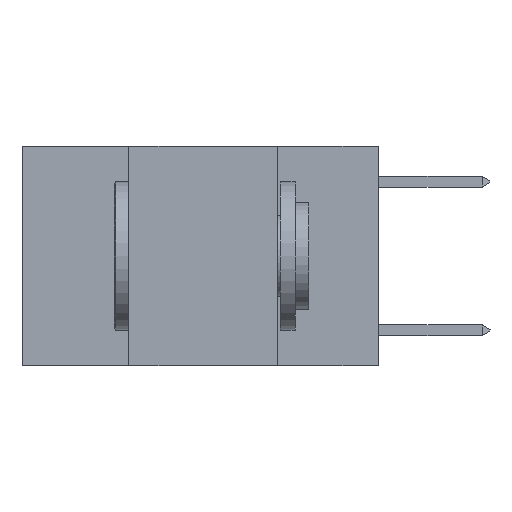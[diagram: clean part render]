
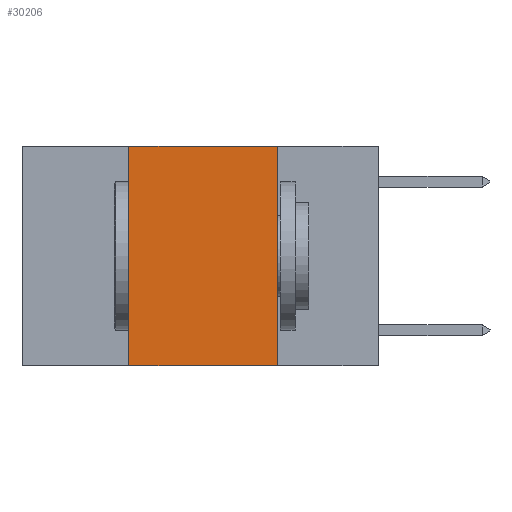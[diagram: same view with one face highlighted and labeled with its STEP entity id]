
A CAD part, left-side view. The second image highlights one B-rep face of the part: STEP entity #30206.
In plain terms, the highlighted planar face has unit normal (-1, 0, 0).
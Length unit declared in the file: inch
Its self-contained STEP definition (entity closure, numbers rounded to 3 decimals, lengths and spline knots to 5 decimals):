
#534 = CARTESIAN_POINT ( 'NONE',  ( 0., 0.6, 0. ) ) ;
#1470 = DIRECTION ( 'NONE',  ( 0., 0., 1. ) ) ;
#2438 = CARTESIAN_POINT ( 'NONE',  ( 0., 0.17, 0. ) ) ;
#2577 = EDGE_LOOP ( 'NONE', ( #27407, #30141, #26272, #7437 ) ) ;
#2658 = PLANE ( 'NONE',  #6689 ) ;
#3578 = VERTEX_POINT ( 'NONE', #10964 ) ;
#3773 = VECTOR ( 'NONE', #1470, 39.37008 ) ;
#6465 = LINE ( 'NONE', #16656, #3773 ) ;
#6689 = AXIS2_PLACEMENT_3D ( 'NONE', #15357, #28516, #30994 ) ;
#7437 = ORIENTED_EDGE ( 'NONE', *, *, #11420, .T. ) ;
#10178 = FACE_OUTER_BOUND ( 'NONE', #2577, .T. ) ;
#10964 = CARTESIAN_POINT ( 'NONE',  ( 0., 0.17, 0. ) ) ;
#10975 = VERTEX_POINT ( 'NONE', #28634 ) ;
#11420 = EDGE_CURVE ( 'NONE', #10975, #32521, #25782, .T. ) ;
#11458 = VECTOR ( 'NONE', #25493, 39.37008 ) ;
#12229 = EDGE_CURVE ( 'NONE', #3578, #32521, #30315, .T. ) ;
#12415 = CARTESIAN_POINT ( 'NONE',  ( 0., 0.42, 0. ) ) ;
#13580 = CARTESIAN_POINT ( 'NONE',  ( 0., 0.6, -0.37 ) ) ;
#15357 = CARTESIAN_POINT ( 'NONE',  ( 0., 0.6, 0. ) ) ;
#15565 = LINE ( 'NONE', #534, #17685 ) ;
#16656 = CARTESIAN_POINT ( 'NONE',  ( 0., 0.42, 0. ) ) ;
#17685 = VECTOR ( 'NONE', #20249, 39.37008 ) ;
#20249 = DIRECTION ( 'NONE',  ( 0., -1., 0. ) ) ;
#23158 = EDGE_CURVE ( 'NONE', #10975, #25238, #6465, .T. ) ;
#24040 = EDGE_CURVE ( 'NONE', #25238, #3578, #15565, .T. ) ;
#24216 = VECTOR ( 'NONE', #26273, 39.37008 ) ;
#25238 = VERTEX_POINT ( 'NONE', #12415 ) ;
#25493 = DIRECTION ( 'NONE',  ( 0., 0., -1. ) ) ;
#25782 = LINE ( 'NONE', #13580, #24216 ) ;
#26272 = ORIENTED_EDGE ( 'NONE', *, *, #23158, .F. ) ;
#26273 = DIRECTION ( 'NONE',  ( 0., -1., 0. ) ) ;
#27407 = ORIENTED_EDGE ( 'NONE', *, *, #12229, .F. ) ;
#28516 = DIRECTION ( 'NONE',  ( 1., 0., 0. ) ) ;
#28634 = CARTESIAN_POINT ( 'NONE',  ( 0., 0.42, -0.37 ) ) ;
#29316 = CARTESIAN_POINT ( 'NONE',  ( 0., 0.17, -0.37 ) ) ;
#30141 = ORIENTED_EDGE ( 'NONE', *, *, #24040, .F. ) ;
#30206 = ADVANCED_FACE ( 'NONE', ( #10178 ), #2658, .F. ) ;
#30315 = LINE ( 'NONE', #2438, #11458 ) ;
#30994 = DIRECTION ( 'NONE',  ( 0., 0., -1. ) ) ;
#32521 = VERTEX_POINT ( 'NONE', #29316 ) ;
